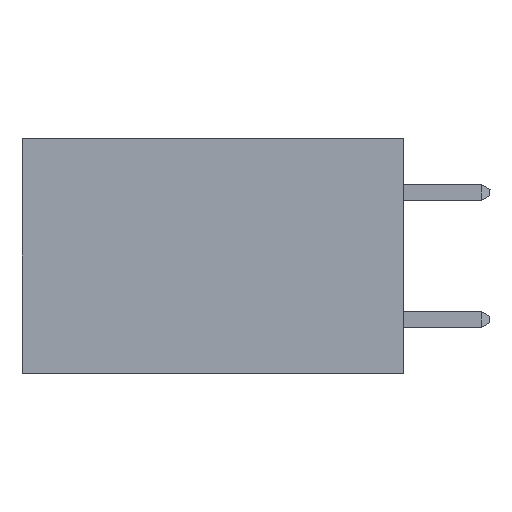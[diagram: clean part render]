
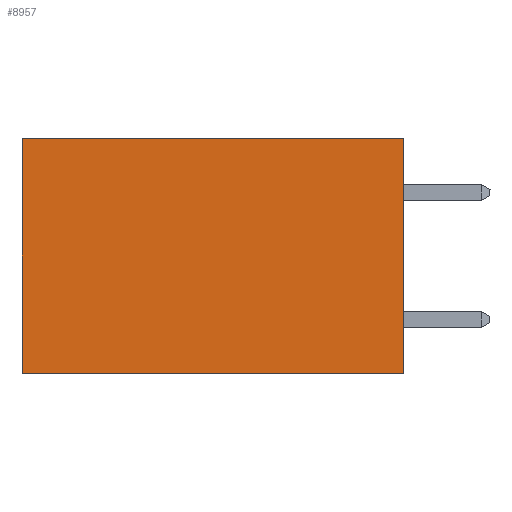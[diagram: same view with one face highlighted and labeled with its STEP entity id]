
A CAD part, left-side view. The second image highlights one B-rep face of the part: STEP entity #8957.
In plain terms, the highlighted planar face has unit normal (-1, 0, 0).
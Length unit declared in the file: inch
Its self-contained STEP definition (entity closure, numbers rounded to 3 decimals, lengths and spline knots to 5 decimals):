
#1697 = DIRECTION ( 'NONE',  ( 0., 0., -1. ) ) ;
#2226 = ORIENTED_EDGE ( 'NONE', *, *, #8575, .T. ) ;
#2581 = CARTESIAN_POINT ( 'NONE',  ( 0.2875, 0., -0.37 ) ) ;
#3199 = CARTESIAN_POINT ( 'NONE',  ( 0.2875, 0., 0. ) ) ;
#3818 = ORIENTED_EDGE ( 'NONE', *, *, #9821, .F. ) ;
#5216 = CARTESIAN_POINT ( 'NONE',  ( 0.2875, 0., 0. ) ) ;
#6964 = VERTEX_POINT ( 'NONE', #2581 ) ;
#7587 = VECTOR ( 'NONE', #12685, 39.37008 ) ;
#7625 = CARTESIAN_POINT ( 'NONE',  ( 0.2875, 0.6, 0. ) ) ;
#8575 = EDGE_CURVE ( 'NONE', #17139, #23347, #25353, .T. ) ;
#8957 = ADVANCED_FACE ( 'NONE', ( #21519 ), #12749, .F. ) ;
#9731 = ORIENTED_EDGE ( 'NONE', *, *, #16447, .F. ) ;
#9821 = EDGE_CURVE ( 'NONE', #6964, #23347, #10255, .T. ) ;
#9926 = LINE ( 'NONE', #12674, #21116 ) ;
#10255 = LINE ( 'NONE', #13389, #26647 ) ;
#12674 = CARTESIAN_POINT ( 'NONE',  ( 0.2875, 0., 0. ) ) ;
#12685 = DIRECTION ( 'NONE',  ( 0., 0., -1. ) ) ;
#12749 = PLANE ( 'NONE',  #27627 ) ;
#13042 = ORIENTED_EDGE ( 'NONE', *, *, #27672, .T. ) ;
#13389 = CARTESIAN_POINT ( 'NONE',  ( 0.2875, 0., -0.37 ) ) ;
#13484 = CARTESIAN_POINT ( 'NONE',  ( 0.2875, 0.6, -0.37 ) ) ;
#14992 = DIRECTION ( 'NONE',  ( 1., 0., 0. ) ) ;
#16447 = EDGE_CURVE ( 'NONE', #18999, #6964, #23292, .T. ) ;
#17139 = VERTEX_POINT ( 'NONE', #7625 ) ;
#18999 = VERTEX_POINT ( 'NONE', #5216 ) ;
#19387 = CARTESIAN_POINT ( 'NONE',  ( 0.2875, 0., 0. ) ) ;
#19412 = DIRECTION ( 'NONE',  ( 0., 1., 0. ) ) ;
#21009 = DIRECTION ( 'NONE',  ( 0., 0., -1. ) ) ;
#21116 = VECTOR ( 'NONE', #19412, 39.37008 ) ;
#21519 = FACE_OUTER_BOUND ( 'NONE', #22728, .T. ) ;
#22293 = DIRECTION ( 'NONE',  ( 0., 1., 0. ) ) ;
#22728 = EDGE_LOOP ( 'NONE', ( #2226, #3818, #9731, #13042 ) ) ;
#23292 = LINE ( 'NONE', #3199, #28480 ) ;
#23347 = VERTEX_POINT ( 'NONE', #13484 ) ;
#25353 = LINE ( 'NONE', #28278, #7587 ) ;
#26647 = VECTOR ( 'NONE', #22293, 39.37008 ) ;
#27627 = AXIS2_PLACEMENT_3D ( 'NONE', #19387, #14992, #1697 ) ;
#27672 = EDGE_CURVE ( 'NONE', #18999, #17139, #9926, .T. ) ;
#28278 = CARTESIAN_POINT ( 'NONE',  ( 0.2875, 0.6, 0. ) ) ;
#28480 = VECTOR ( 'NONE', #21009, 39.37008 ) ;
